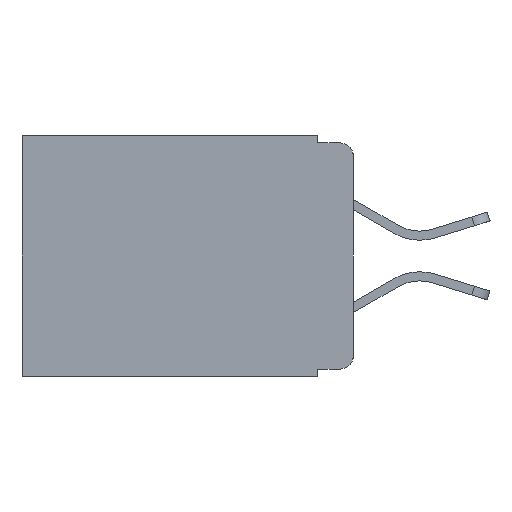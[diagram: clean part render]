
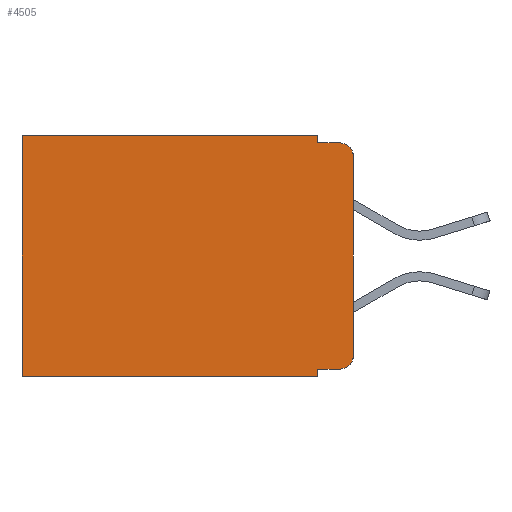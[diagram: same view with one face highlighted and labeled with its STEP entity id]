
A CAD part, left-side view. The second image highlights one B-rep face of the part: STEP entity #4505.
In plain terms, the highlighted planar face has unit normal (-1, 0, 0).
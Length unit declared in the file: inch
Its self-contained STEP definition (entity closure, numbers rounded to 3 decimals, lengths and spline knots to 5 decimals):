
#70 = ORIENTED_EDGE ( 'NONE', *, *, #9495, .T. ) ;
#91 = LINE ( 'NONE', #10268, #7595 ) ;
#105 = LINE ( 'NONE', #7553, #2824 ) ;
#157 = ORIENTED_EDGE ( 'NONE', *, *, #10047, .T. ) ;
#443 = ORIENTED_EDGE ( 'NONE', *, *, #11405, .F. ) ;
#468 = DIRECTION ( 'NONE',  ( 0., 0., -1. ) ) ;
#596 = CARTESIAN_POINT ( 'NONE',  ( 0.298, 0.051, -0.343 ) ) ;
#684 = CARTESIAN_POINT ( 'NONE',  ( 0.298, 0., -0.03 ) ) ;
#692 = ORIENTED_EDGE ( 'NONE', *, *, #737, .T. ) ;
#737 = EDGE_CURVE ( 'NONE', #8172, #1902, #7762, .T. ) ;
#825 = ORIENTED_EDGE ( 'NONE', *, *, #10580, .F. ) ;
#1062 = ORIENTED_EDGE ( 'NONE', *, *, #3994, .F. ) ;
#1109 = EDGE_CURVE ( 'NONE', #4068, #8172, #6798, .T. ) ;
#1260 = CARTESIAN_POINT ( 'NONE',  ( 0.298, 0.051, 0. ) ) ;
#1279 = VERTEX_POINT ( 'NONE', #7120 ) ;
#1309 = DIRECTION ( 'NONE',  ( 0., -1., 0. ) ) ;
#1394 = VERTEX_POINT ( 'NONE', #7470 ) ;
#1422 = EDGE_CURVE ( 'NONE', #4068, #9624, #11093, .T. ) ;
#1470 = ORIENTED_EDGE ( 'NONE', *, *, #1109, .T. ) ;
#1570 = VECTOR ( 'NONE', #10591, 39.37008 ) ;
#1589 = VECTOR ( 'NONE', #7534, 39.37008 ) ;
#1590 = CIRCLE ( 'NONE', #8691, 0.02 ) ;
#1902 = VERTEX_POINT ( 'NONE', #2999 ) ;
#2007 = CARTESIAN_POINT ( 'NONE',  ( 0.298, 0.02, -0.01 ) ) ;
#2097 = EDGE_CURVE ( 'NONE', #9624, #3503, #6241, .T. ) ;
#2120 = CARTESIAN_POINT ( 'NONE',  ( 0.298, 0.051, -0.01 ) ) ;
#2354 = CARTESIAN_POINT ( 'NONE',  ( 0.298, 0.051, 0. ) ) ;
#2470 = ORIENTED_EDGE ( 'NONE', *, *, #2762, .T. ) ;
#2503 = AXIS2_PLACEMENT_3D ( 'NONE', #11052, #4917, #4945 ) ;
#2562 = AXIS2_PLACEMENT_3D ( 'NONE', #3816, #3585, #4565 ) ;
#2762 = EDGE_CURVE ( 'NONE', #8371, #3503, #6902, .T. ) ;
#2824 = VECTOR ( 'NONE', #3161, 39.37008 ) ;
#2999 = CARTESIAN_POINT ( 'NONE',  ( 0.298, 0.473, -0.343 ) ) ;
#3161 = DIRECTION ( 'NONE',  ( 0., 0., -1. ) ) ;
#3503 = VERTEX_POINT ( 'NONE', #2007 ) ;
#3585 = DIRECTION ( 'NONE',  ( -1., 0., 0. ) ) ;
#3816 = CARTESIAN_POINT ( 'NONE',  ( 0.298, 0.02, -0.03 ) ) ;
#3994 = EDGE_CURVE ( 'NONE', #8371, #1394, #105, .T. ) ;
#4022 = ORIENTED_EDGE ( 'NONE', *, *, #2097, .F. ) ;
#4068 = VERTEX_POINT ( 'NONE', #2354 ) ;
#4193 = CARTESIAN_POINT ( 'NONE',  ( 0.298, 0., 0. ) ) ;
#4269 = VECTOR ( 'NONE', #5952, 39.37008 ) ;
#4505 = ADVANCED_FACE ( 'NONE', ( #6911 ), #5075, .F. ) ;
#4565 = DIRECTION ( 'NONE',  ( 0., 0., -1. ) ) ;
#4917 = DIRECTION ( 'NONE',  ( 1., 0., 0. ) ) ;
#4945 = DIRECTION ( 'NONE',  ( 0., 0., -1. ) ) ;
#5064 = CARTESIAN_POINT ( 'NONE',  ( 0.298, 0.051, 0. ) ) ;
#5075 = PLANE ( 'NONE',  #2503 ) ;
#5476 = EDGE_LOOP ( 'NONE', ( #1062, #2470, #4022, #8139, #1470, #692, #443, #825, #157, #70 ) ) ;
#5551 = VERTEX_POINT ( 'NONE', #596 ) ;
#5952 = DIRECTION ( 'NONE',  ( 0., 0., -1. ) ) ;
#6168 = DIRECTION ( 'NONE',  ( -1., 0., 0. ) ) ;
#6241 = LINE ( 'NONE', #2120, #1570 ) ;
#6661 = VECTOR ( 'NONE', #7253, 39.37008 ) ;
#6798 = LINE ( 'NONE', #4193, #1589 ) ;
#6902 = CIRCLE ( 'NONE', #2562, 0.02 ) ;
#6911 = FACE_OUTER_BOUND ( 'NONE', #5476, .T. ) ;
#6927 = VECTOR ( 'NONE', #1309, 39.37008 ) ;
#7120 = CARTESIAN_POINT ( 'NONE',  ( 0.298, 0.051, -0.333 ) ) ;
#7224 = CARTESIAN_POINT ( 'NONE',  ( 0.298, 0.051, -0.01 ) ) ;
#7253 = DIRECTION ( 'NONE',  ( 0., 0., -1. ) ) ;
#7470 = CARTESIAN_POINT ( 'NONE',  ( 0.298, 0., -0.313 ) ) ;
#7534 = DIRECTION ( 'NONE',  ( 0., 1., 0. ) ) ;
#7553 = CARTESIAN_POINT ( 'NONE',  ( 0.298, 0., 0. ) ) ;
#7595 = VECTOR ( 'NONE', #11073, 39.37008 ) ;
#7716 = CARTESIAN_POINT ( 'NONE',  ( 0.298, 0.473, 0. ) ) ;
#7762 = LINE ( 'NONE', #9686, #9723 ) ;
#8139 = ORIENTED_EDGE ( 'NONE', *, *, #1422, .F. ) ;
#8172 = VERTEX_POINT ( 'NONE', #7716 ) ;
#8371 = VERTEX_POINT ( 'NONE', #684 ) ;
#8691 = AXIS2_PLACEMENT_3D ( 'NONE', #11165, #6168, #468 ) ;
#8917 = LINE ( 'NONE', #1260, #4269 ) ;
#9195 = LINE ( 'NONE', #10226, #6927 ) ;
#9495 = EDGE_CURVE ( 'NONE', #10773, #1394, #1590, .T. ) ;
#9624 = VERTEX_POINT ( 'NONE', #7224 ) ;
#9686 = CARTESIAN_POINT ( 'NONE',  ( 0.298, 0.473, 0. ) ) ;
#9723 = VECTOR ( 'NONE', #10630, 39.37008 ) ;
#10047 = EDGE_CURVE ( 'NONE', #1279, #10773, #9195, .T. ) ;
#10226 = CARTESIAN_POINT ( 'NONE',  ( 0.298, 0.051, -0.333 ) ) ;
#10268 = CARTESIAN_POINT ( 'NONE',  ( 0.298, 0., -0.343 ) ) ;
#10424 = CARTESIAN_POINT ( 'NONE',  ( 0.298, 0.02, -0.333 ) ) ;
#10580 = EDGE_CURVE ( 'NONE', #1279, #5551, #8917, .T. ) ;
#10591 = DIRECTION ( 'NONE',  ( 0., -1., 0. ) ) ;
#10630 = DIRECTION ( 'NONE',  ( 0., 0., -1. ) ) ;
#10773 = VERTEX_POINT ( 'NONE', #10424 ) ;
#11052 = CARTESIAN_POINT ( 'NONE',  ( 0.298, 0., 0. ) ) ;
#11073 = DIRECTION ( 'NONE',  ( 0., 1., 0. ) ) ;
#11093 = LINE ( 'NONE', #5064, #6661 ) ;
#11165 = CARTESIAN_POINT ( 'NONE',  ( 0.298, 0.02, -0.313 ) ) ;
#11405 = EDGE_CURVE ( 'NONE', #5551, #1902, #91, .T. ) ;
